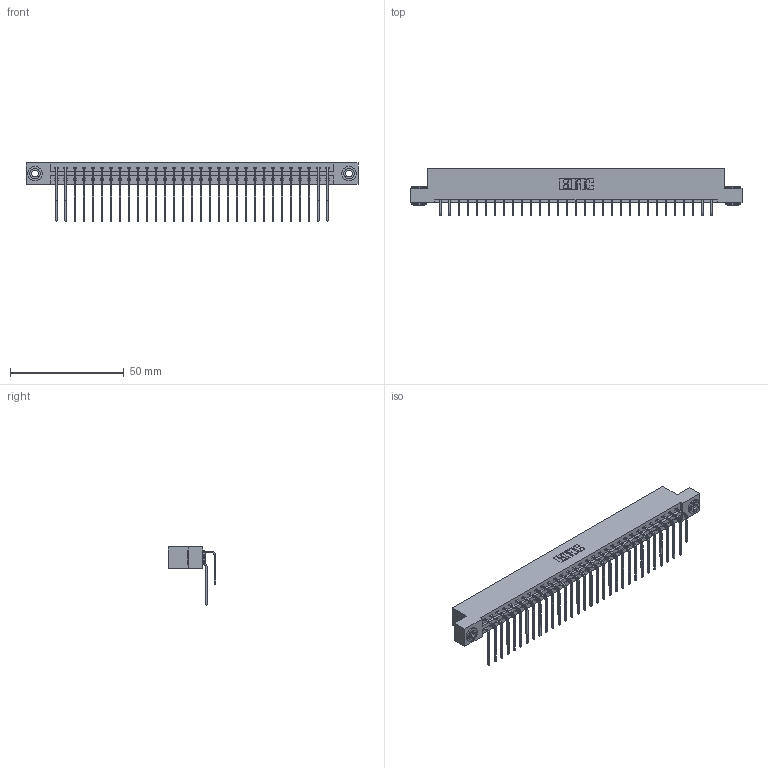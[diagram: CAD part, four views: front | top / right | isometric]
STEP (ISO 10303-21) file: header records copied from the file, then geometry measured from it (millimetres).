
FILE_DESCRIPTION (( 'STEP AP203' ), '1' );
FILE_NAME ('387-062-559-203.STEP', '2019-10-19T15:48:28', ( '' ), ( '' ), 'SwSTEP 2.0', 'SolidWorks 2016', '' );
FILE_SCHEMA (( 'CONFIG_CONTROL_DESIGN' ));
Length unit declared in the file: inch
Products named in the file (5): 345-292-001_558 559 Tail - 1; 345-250-002_345-250-002-102; 387-062-559-203; 345-292-001_559 Tail - 2; 337 Part_Flush Mounting Lugs - 0.156 Dia-TH
Assembly tree (65 placements, depth 2):
  387-062-559-203
    337 Part_Flush Mounting Lugs - 0.156 Dia-TH
    345-292-001_558 559 Tail - 1  x31
    345-292-001_559 Tail - 2  x31
    345-250-002_345-250-002-102  x2
Bounding box: 145.85 x 20.9 x 25.53 mm (x, y, z)
Volume: 15601.1 mm3; surface area: 19550.6 mm2
Topology: 65 solids, 65 shells, 3624 faces, 10741 edges, 7074 vertices
Faces by surface type: plane 2560, cylinder 1056, cone 8
Entity records: 27892 total; most frequent: CARTESIAN_POINT 4728, ORIENTED_EDGE 4606, DIRECTION 4057, EDGE_CURVE 2303, LINE 2111, VECTOR 2111, VERTEX_POINT 1530, AXIS2_PLACEMENT_3D 973
